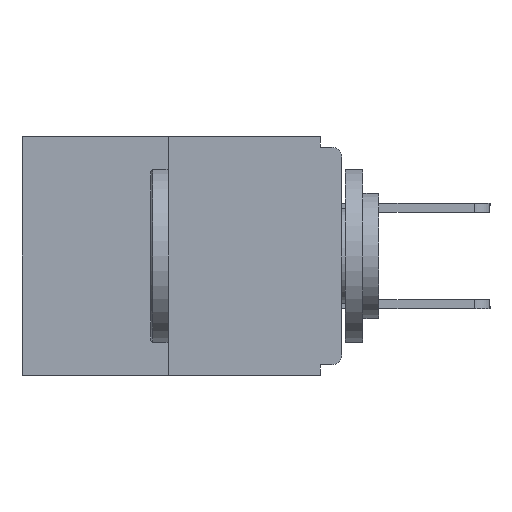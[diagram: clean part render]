
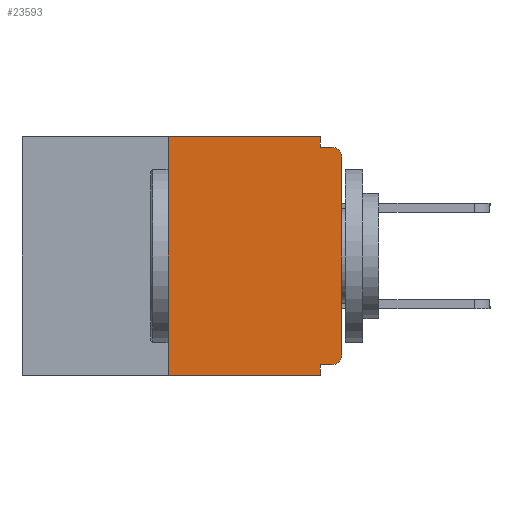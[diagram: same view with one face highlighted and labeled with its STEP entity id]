
A CAD part, left-side view. The second image highlights one B-rep face of the part: STEP entity #23593.
In plain terms, the highlighted planar face has unit normal (-1, 0, 0).
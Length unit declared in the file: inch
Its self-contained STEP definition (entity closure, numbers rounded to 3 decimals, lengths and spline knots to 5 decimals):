
#442 = CARTESIAN_POINT ( 'NONE',  ( 0., 0., -0.328 ) ) ;
#944 = EDGE_CURVE ( 'NONE', #9411, #24369, #13651, .T. ) ;
#1388 = CARTESIAN_POINT ( 'NONE',  ( 0., 0.031, -0.343 ) ) ;
#1548 = AXIS2_PLACEMENT_3D ( 'NONE', #1587, #11530, #23147 ) ;
#1587 = CARTESIAN_POINT ( 'NONE',  ( 0., 0.015, -0.03 ) ) ;
#1762 = CIRCLE ( 'NONE', #25202, 0.015 ) ;
#2190 = VECTOR ( 'NONE', #25249, 39.37008 ) ;
#3610 = LINE ( 'NONE', #1388, #3960 ) ;
#3960 = VECTOR ( 'NONE', #13439, 39.37008 ) ;
#4108 = LINE ( 'NONE', #19451, #15769 ) ;
#4262 = ORIENTED_EDGE ( 'NONE', *, *, #944, .F. ) ;
#6540 = CARTESIAN_POINT ( 'NONE',  ( 0., 0.46, -0.343 ) ) ;
#6575 = VERTEX_POINT ( 'NONE', #11583 ) ;
#7275 = VERTEX_POINT ( 'NONE', #17471 ) ;
#7709 = LINE ( 'NONE', #6540, #26094 ) ;
#7906 = ORIENTED_EDGE ( 'NONE', *, *, #27227, .F. ) ;
#8849 = LINE ( 'NONE', #13140, #28718 ) ;
#9411 = VERTEX_POINT ( 'NONE', #17031 ) ;
#10683 = EDGE_CURVE ( 'NONE', #29546, #19422, #29827, .T. ) ;
#10786 = LINE ( 'NONE', #27877, #2190 ) ;
#11262 = CARTESIAN_POINT ( 'NONE',  ( 0., 0., 0. ) ) ;
#11423 = DIRECTION ( 'NONE',  ( 0., 0., -1. ) ) ;
#11530 = DIRECTION ( 'NONE',  ( -1., 0., 0. ) ) ;
#11583 = CARTESIAN_POINT ( 'NONE',  ( 0., 0.031, -0.015 ) ) ;
#11822 = CARTESIAN_POINT ( 'NONE',  ( 0., 0.25, 0. ) ) ;
#12081 = ORIENTED_EDGE ( 'NONE', *, *, #28761, .F. ) ;
#12540 = ORIENTED_EDGE ( 'NONE', *, *, #10683, .T. ) ;
#12567 = DIRECTION ( 'NONE',  ( 0., 1., 0. ) ) ;
#13140 = CARTESIAN_POINT ( 'NONE',  ( 0., 0., -0.015 ) ) ;
#13439 = DIRECTION ( 'NONE',  ( 0., 0., -1. ) ) ;
#13465 = DIRECTION ( 'NONE',  ( 0., -1., 0. ) ) ;
#13651 = LINE ( 'NONE', #442, #15516 ) ;
#14357 = PLANE ( 'NONE',  #24395 ) ;
#14952 = EDGE_CURVE ( 'NONE', #9411, #29546, #1762, .T. ) ;
#14960 = EDGE_CURVE ( 'NONE', #19422, #22837, #26147, .T. ) ;
#15340 = DIRECTION ( 'NONE',  ( 0., 0., 1. ) ) ;
#15516 = VECTOR ( 'NONE', #12567, 39.37008 ) ;
#15769 = VECTOR ( 'NONE', #26393, 39.37008 ) ;
#16189 = DIRECTION ( 'NONE',  ( 0., -1., 0. ) ) ;
#16277 = VERTEX_POINT ( 'NONE', #17258 ) ;
#17031 = CARTESIAN_POINT ( 'NONE',  ( 0., 0.015, -0.328 ) ) ;
#17258 = CARTESIAN_POINT ( 'NONE',  ( 0., 0.031, 0. ) ) ;
#17471 = CARTESIAN_POINT ( 'NONE',  ( 0., 0.031, -0.343 ) ) ;
#17651 = VERTEX_POINT ( 'NONE', #26142 ) ;
#18005 = EDGE_CURVE ( 'NONE', #17651, #29225, #28941, .T. ) ;
#18444 = CARTESIAN_POINT ( 'NONE',  ( 0., 0.015, -0.015 ) ) ;
#18604 = CARTESIAN_POINT ( 'NONE',  ( 0., 0., -0.03 ) ) ;
#18623 = CARTESIAN_POINT ( 'NONE',  ( 0., 0.031, -0.328 ) ) ;
#19422 = VERTEX_POINT ( 'NONE', #18604 ) ;
#19451 = CARTESIAN_POINT ( 'NONE',  ( 0., 0.031, 0. ) ) ;
#19841 = EDGE_CURVE ( 'NONE', #16277, #6575, #4108, .T. ) ;
#20115 = ORIENTED_EDGE ( 'NONE', *, *, #19841, .F. ) ;
#20956 = CARTESIAN_POINT ( 'NONE',  ( 0., 0.015, -0.313 ) ) ;
#21229 = ORIENTED_EDGE ( 'NONE', *, *, #18005, .F. ) ;
#21578 = EDGE_LOOP ( 'NONE', ( #7906, #21229, #22921, #25678, #4262, #25541, #12540, #25622, #12081, #20115 ) ) ;
#21679 = EDGE_CURVE ( 'NONE', #24369, #7275, #3610, .T. ) ;
#22183 = EDGE_CURVE ( 'NONE', #17651, #7275, #7709, .T. ) ;
#22452 = CARTESIAN_POINT ( 'NONE',  ( 0., 0.25, 0. ) ) ;
#22837 = VERTEX_POINT ( 'NONE', #18444 ) ;
#22921 = ORIENTED_EDGE ( 'NONE', *, *, #22183, .T. ) ;
#22956 = VECTOR ( 'NONE', #15340, 39.37008 ) ;
#23147 = DIRECTION ( 'NONE',  ( 0., 0., -1. ) ) ;
#23593 = ADVANCED_FACE ( 'NONE', ( #28276 ), #14357, .F. ) ;
#23976 = DIRECTION ( 'NONE',  ( 1., 0., 0. ) ) ;
#24369 = VERTEX_POINT ( 'NONE', #18623 ) ;
#24395 = AXIS2_PLACEMENT_3D ( 'NONE', #31064, #23976, #26483 ) ;
#25202 = AXIS2_PLACEMENT_3D ( 'NONE', #20956, #28174, #11423 ) ;
#25249 = DIRECTION ( 'NONE',  ( 0., -1., 0. ) ) ;
#25541 = ORIENTED_EDGE ( 'NONE', *, *, #14952, .T. ) ;
#25622 = ORIENTED_EDGE ( 'NONE', *, *, #14960, .T. ) ;
#25678 = ORIENTED_EDGE ( 'NONE', *, *, #21679, .F. ) ;
#26094 = VECTOR ( 'NONE', #16189, 39.37008 ) ;
#26142 = CARTESIAN_POINT ( 'NONE',  ( 0., 0.25, -0.343 ) ) ;
#26147 = CIRCLE ( 'NONE', #1548, 0.015 ) ;
#26393 = DIRECTION ( 'NONE',  ( 0., 0., -1. ) ) ;
#26483 = DIRECTION ( 'NONE',  ( 0., 0., -1. ) ) ;
#27227 = EDGE_CURVE ( 'NONE', #29225, #16277, #10786, .T. ) ;
#27877 = CARTESIAN_POINT ( 'NONE',  ( 0., 0.46, 0. ) ) ;
#28174 = DIRECTION ( 'NONE',  ( -1., 0., 0. ) ) ;
#28276 = FACE_OUTER_BOUND ( 'NONE', #21578, .T. ) ;
#28327 = VECTOR ( 'NONE', #30243, 39.37008 ) ;
#28698 = CARTESIAN_POINT ( 'NONE',  ( 0., 0., -0.313 ) ) ;
#28718 = VECTOR ( 'NONE', #13465, 39.37008 ) ;
#28761 = EDGE_CURVE ( 'NONE', #6575, #22837, #8849, .T. ) ;
#28941 = LINE ( 'NONE', #22452, #22956 ) ;
#29225 = VERTEX_POINT ( 'NONE', #11822 ) ;
#29546 = VERTEX_POINT ( 'NONE', #28698 ) ;
#29827 = LINE ( 'NONE', #11262, #28327 ) ;
#30243 = DIRECTION ( 'NONE',  ( 0., 0., 1. ) ) ;
#31064 = CARTESIAN_POINT ( 'NONE',  ( 0., 0.46, 0. ) ) ;
